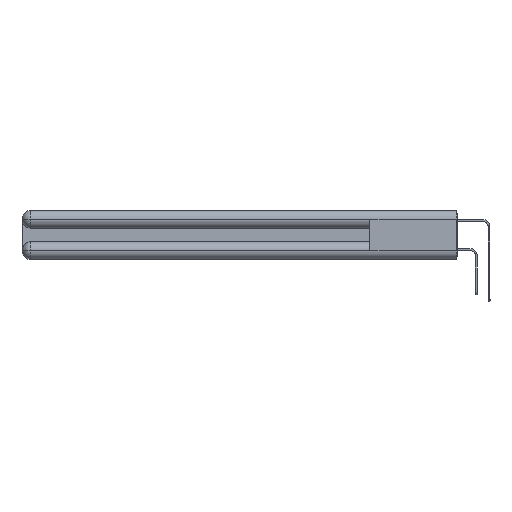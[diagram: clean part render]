
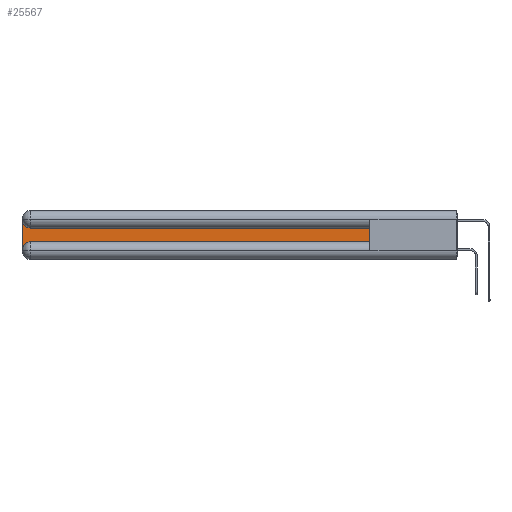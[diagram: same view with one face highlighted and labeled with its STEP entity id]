
A CAD part, left-side view. The second image highlights one B-rep face of the part: STEP entity #25567.
In plain terms, the highlighted planar face has unit normal (-1, 0, 0).
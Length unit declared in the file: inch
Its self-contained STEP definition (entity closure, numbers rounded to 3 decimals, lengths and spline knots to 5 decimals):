
#97 = EDGE_CURVE ( 'NONE', #28758, #6620, #15683, .T. ) ;
#144 = AXIS2_PLACEMENT_3D ( 'NONE', #25408, #11657, #5162 ) ;
#182 = DIRECTION ( 'NONE',  ( 0., -1., 0. ) ) ;
#1321 = DIRECTION ( 'NONE',  ( 0., 0., -1. ) ) ;
#1741 = EDGE_LOOP ( 'NONE', ( #11822, #6308, #13661, #22962, #9227, #2100 ) ) ;
#2100 = ORIENTED_EDGE ( 'NONE', *, *, #16052, .T. ) ;
#2366 = DIRECTION ( 'NONE',  ( 0., 0., 1. ) ) ;
#2424 = EDGE_CURVE ( 'NONE', #21691, #28758, #6965, .T. ) ;
#2945 = AXIS2_PLACEMENT_3D ( 'NONE', #6958, #4594, #27061 ) ;
#3082 = CARTESIAN_POINT ( 'NONE',  ( 0.075, 0.6, -0.2175 ) ) ;
#4594 = DIRECTION ( 'NONE',  ( 1., 0., 0. ) ) ;
#5162 = DIRECTION ( 'NONE',  ( 0., 0., -1. ) ) ;
#5421 = CARTESIAN_POINT ( 'NONE',  ( 0.075, 2.94, -0.2775 ) ) ;
#6308 = ORIENTED_EDGE ( 'NONE', *, *, #97, .T. ) ;
#6620 = VERTEX_POINT ( 'NONE', #12823 ) ;
#6958 = CARTESIAN_POINT ( 'NONE',  ( 0.075, 2.94, -0.0625 ) ) ;
#6965 = LINE ( 'NONE', #21007, #18796 ) ;
#7881 = VECTOR ( 'NONE', #182, 39.37008 ) ;
#9227 = ORIENTED_EDGE ( 'NONE', *, *, #20237, .T. ) ;
#9618 = DIRECTION ( 'NONE',  ( 0., 1., 0. ) ) ;
#11336 = CARTESIAN_POINT ( 'NONE',  ( 0.075, 0.6, -0.2175 ) ) ;
#11657 = DIRECTION ( 'NONE',  ( 1., 0., 0. ) ) ;
#11822 = ORIENTED_EDGE ( 'NONE', *, *, #2424, .T. ) ;
#12087 = VECTOR ( 'NONE', #2366, 39.37008 ) ;
#12140 = CARTESIAN_POINT ( 'NONE',  ( 0.075, 3., -0.2175 ) ) ;
#12823 = CARTESIAN_POINT ( 'NONE',  ( 0.075, 3., -0.0625 ) ) ;
#13661 = ORIENTED_EDGE ( 'NONE', *, *, #15234, .T. ) ;
#13997 = LINE ( 'NONE', #11336, #12087 ) ;
#14600 = DIRECTION ( 'NONE',  ( 1., 0., 0. ) ) ;
#15234 = EDGE_CURVE ( 'NONE', #6620, #26400, #16743, .T. ) ;
#15683 = CIRCLE ( 'NONE', #2945, 0.06 ) ;
#16052 = EDGE_CURVE ( 'NONE', #16169, #21691, #13997, .T. ) ;
#16169 = VERTEX_POINT ( 'NONE', #3082 ) ;
#16413 = PLANE ( 'NONE',  #144 ) ;
#16575 = LINE ( 'NONE', #25424, #7881 ) ;
#16743 = LINE ( 'NONE', #12140, #27255 ) ;
#17310 = AXIS2_PLACEMENT_3D ( 'NONE', #5421, #14600, #1321 ) ;
#17449 = EDGE_CURVE ( 'NONE', #26400, #21350, #22939, .T. ) ;
#18338 = FACE_OUTER_BOUND ( 'NONE', #1741, .T. ) ;
#18680 = CARTESIAN_POINT ( 'NONE',  ( 0.075, 2.94, -0.1225 ) ) ;
#18796 = VECTOR ( 'NONE', #9618, 39.37008 ) ;
#20237 = EDGE_CURVE ( 'NONE', #21350, #16169, #16575, .T. ) ;
#21007 = CARTESIAN_POINT ( 'NONE',  ( 0.075, 0.6, -0.1225 ) ) ;
#21350 = VERTEX_POINT ( 'NONE', #27210 ) ;
#21691 = VERTEX_POINT ( 'NONE', #28528 ) ;
#22939 = CIRCLE ( 'NONE', #17310, 0.06 ) ;
#22962 = ORIENTED_EDGE ( 'NONE', *, *, #17449, .T. ) ;
#25408 = CARTESIAN_POINT ( 'NONE',  ( 0.075, 3., -0.1225 ) ) ;
#25424 = CARTESIAN_POINT ( 'NONE',  ( 0.075, 0.6, -0.2175 ) ) ;
#25567 = ADVANCED_FACE ( 'NONE', ( #18338 ), #16413, .F. ) ;
#26400 = VERTEX_POINT ( 'NONE', #27117 ) ;
#27061 = DIRECTION ( 'NONE',  ( 0., 0., -1. ) ) ;
#27117 = CARTESIAN_POINT ( 'NONE',  ( 0.075, 3., -0.2775 ) ) ;
#27210 = CARTESIAN_POINT ( 'NONE',  ( 0.075, 2.94, -0.2175 ) ) ;
#27255 = VECTOR ( 'NONE', #28401, 39.37008 ) ;
#28401 = DIRECTION ( 'NONE',  ( 0., 0., -1. ) ) ;
#28528 = CARTESIAN_POINT ( 'NONE',  ( 0.075, 0.6, -0.1225 ) ) ;
#28758 = VERTEX_POINT ( 'NONE', #18680 ) ;
